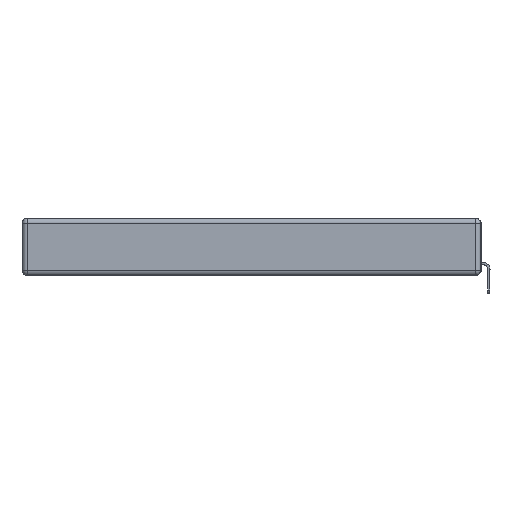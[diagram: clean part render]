
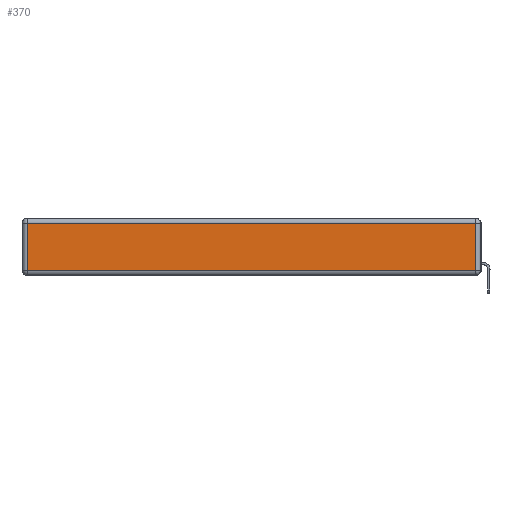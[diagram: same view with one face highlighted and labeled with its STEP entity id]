
A CAD part, left-side view. The second image highlights one B-rep face of the part: STEP entity #370.
In plain terms, the highlighted planar face has unit normal (-1, 0, 0).
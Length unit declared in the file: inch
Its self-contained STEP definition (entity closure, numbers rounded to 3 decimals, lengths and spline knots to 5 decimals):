
#370 = ADVANCED_FACE ( 'NONE', ( #20521 ), #18970, .T. ) ;
#1534 = VECTOR ( 'NONE', #13832, 39.37008 ) ;
#1615 = DIRECTION ( 'NONE',  ( 0., 0., 1. ) ) ;
#2055 = VECTOR ( 'NONE', #5571, 39.37008 ) ;
#2084 = VERTEX_POINT ( 'NONE', #10751 ) ;
#2320 = CARTESIAN_POINT ( 'NONE',  ( 0., 0., -0.313 ) ) ;
#3039 = ORIENTED_EDGE ( 'NONE', *, *, #7647, .T. ) ;
#4289 = VERTEX_POINT ( 'NONE', #6471 ) ;
#4462 = CARTESIAN_POINT ( 'NONE',  ( 0., 0.03, -0.343 ) ) ;
#4917 = VERTEX_POINT ( 'NONE', #10737 ) ;
#5571 = DIRECTION ( 'NONE',  ( 0., -1., 0. ) ) ;
#6471 = CARTESIAN_POINT ( 'NONE',  ( 0., 2.72, -0.03 ) ) ;
#6682 = EDGE_CURVE ( 'NONE', #4289, #2084, #20300, .T. ) ;
#7339 = CARTESIAN_POINT ( 'NONE',  ( 0., 2.72, -0.343 ) ) ;
#7647 = EDGE_CURVE ( 'NONE', #8740, #4289, #12445, .T. ) ;
#8740 = VERTEX_POINT ( 'NONE', #18177 ) ;
#9901 = LINE ( 'NONE', #2320, #2055 ) ;
#9976 = EDGE_CURVE ( 'NONE', #2084, #4917, #9901, .T. ) ;
#10737 = CARTESIAN_POINT ( 'NONE',  ( 0., 0.03, -0.313 ) ) ;
#10751 = CARTESIAN_POINT ( 'NONE',  ( 0., 2.72, -0.313 ) ) ;
#11008 = DIRECTION ( 'NONE',  ( 0., 1., 0. ) ) ;
#11107 = CARTESIAN_POINT ( 'NONE',  ( 0., 2.75, -0.03 ) ) ;
#12394 = ORIENTED_EDGE ( 'NONE', *, *, #6682, .T. ) ;
#12445 = LINE ( 'NONE', #11107, #19663 ) ;
#13161 = EDGE_LOOP ( 'NONE', ( #15820, #19671, #3039, #12394 ) ) ;
#13832 = DIRECTION ( 'NONE',  ( 0., 0., -1. ) ) ;
#15280 = EDGE_CURVE ( 'NONE', #4917, #8740, #15754, .T. ) ;
#15754 = LINE ( 'NONE', #4462, #18962 ) ;
#15820 = ORIENTED_EDGE ( 'NONE', *, *, #9976, .T. ) ;
#15999 = AXIS2_PLACEMENT_3D ( 'NONE', #17397, #20423, #1615 ) ;
#17397 = CARTESIAN_POINT ( 'NONE',  ( 0., 0., -0.343 ) ) ;
#17412 = DIRECTION ( 'NONE',  ( 0., 0., 1. ) ) ;
#18177 = CARTESIAN_POINT ( 'NONE',  ( 0., 0.03, -0.03 ) ) ;
#18962 = VECTOR ( 'NONE', #17412, 39.37008 ) ;
#18970 = PLANE ( 'NONE',  #15999 ) ;
#19663 = VECTOR ( 'NONE', #11008, 39.37008 ) ;
#19671 = ORIENTED_EDGE ( 'NONE', *, *, #15280, .T. ) ;
#20300 = LINE ( 'NONE', #7339, #1534 ) ;
#20423 = DIRECTION ( 'NONE',  ( -1., 0., 0. ) ) ;
#20521 = FACE_OUTER_BOUND ( 'NONE', #13161, .T. ) ;
